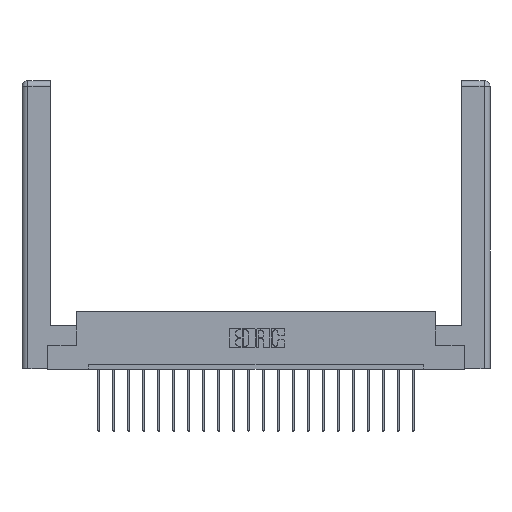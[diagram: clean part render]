
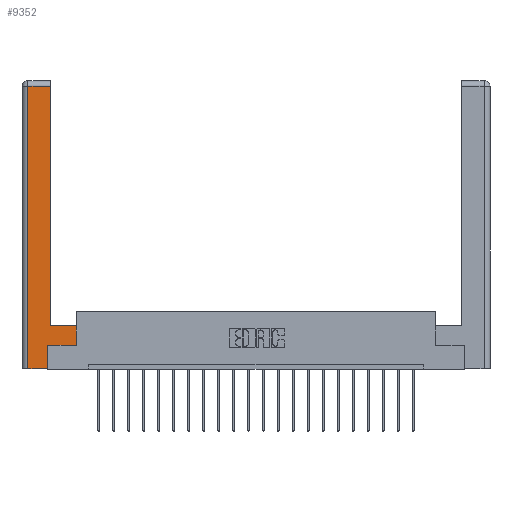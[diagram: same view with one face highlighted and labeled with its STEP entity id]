
A CAD part, top view. The second image highlights one B-rep face of the part: STEP entity #9352.
In plain terms, the highlighted planar face has unit normal (0, 0, 1).
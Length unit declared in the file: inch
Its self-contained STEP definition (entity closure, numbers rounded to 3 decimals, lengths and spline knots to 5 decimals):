
#75 = DIRECTION ( 'NONE',  ( 0., 1., 0. ) ) ;
#248 = VERTEX_POINT ( 'NONE', #835 ) ;
#651 = DIRECTION ( 'NONE',  ( 1., 0., 0. ) ) ;
#835 = CARTESIAN_POINT ( 'NONE',  ( 0.265, 0.245, 0. ) ) ;
#1026 = CARTESIAN_POINT ( 'NONE',  ( 0.295, 3., 0. ) ) ;
#1668 = ORIENTED_EDGE ( 'NONE', *, *, #7298, .T. ) ;
#2332 = CARTESIAN_POINT ( 'NONE',  ( 0.295, 0.45, 0. ) ) ;
#2423 = VERTEX_POINT ( 'NONE', #12963 ) ;
#3326 = CARTESIAN_POINT ( 'NONE',  ( 0.265, 0., 0. ) ) ;
#3584 = LINE ( 'NONE', #17032, #11918 ) ;
#3739 = CARTESIAN_POINT ( 'NONE',  ( 0.0615, 2.94, 0. ) ) ;
#3885 = LINE ( 'NONE', #20429, #16706 ) ;
#3983 = CARTESIAN_POINT ( 'NONE',  ( 0.295, 0.45, 0. ) ) ;
#4080 = ORIENTED_EDGE ( 'NONE', *, *, #11053, .T. ) ;
#4173 = CARTESIAN_POINT ( 'NONE',  ( 0.0615, 0., 0. ) ) ;
#4557 = VECTOR ( 'NONE', #16235, 39.37008 ) ;
#5011 = VERTEX_POINT ( 'NONE', #5076 ) ;
#5012 = CARTESIAN_POINT ( 'NONE',  ( 0., 0., 0. ) ) ;
#5076 = CARTESIAN_POINT ( 'NONE',  ( 0.565, 0.45, 0. ) ) ;
#5267 = AXIS2_PLACEMENT_3D ( 'NONE', #5012, #10126, #20235 ) ;
#5291 = VERTEX_POINT ( 'NONE', #2332 ) ;
#5506 = EDGE_CURVE ( 'NONE', #18912, #248, #3584, .T. ) ;
#5746 = LINE ( 'NONE', #15785, #8893 ) ;
#5751 = DIRECTION ( 'NONE',  ( -1., 0., 0. ) ) ;
#6226 = CARTESIAN_POINT ( 'NONE',  ( 0.0615, 0., 0. ) ) ;
#6699 = LINE ( 'NONE', #6226, #4557 ) ;
#6967 = EDGE_CURVE ( 'NONE', #5011, #5291, #21251, .T. ) ;
#7298 = EDGE_CURVE ( 'NONE', #2423, #18164, #9268, .T. ) ;
#7407 = VECTOR ( 'NONE', #11629, 39.37008 ) ;
#7627 = ORIENTED_EDGE ( 'NONE', *, *, #17752, .T. ) ;
#7664 = ORIENTED_EDGE ( 'NONE', *, *, #5506, .T. ) ;
#8056 = VECTOR ( 'NONE', #17712, 39.37008 ) ;
#8392 = FACE_OUTER_BOUND ( 'NONE', #14338, .T. ) ;
#8604 = LINE ( 'NONE', #1026, #8056 ) ;
#8893 = VECTOR ( 'NONE', #12762, 39.37008 ) ;
#9268 = LINE ( 'NONE', #3739, #15536 ) ;
#9352 = ADVANCED_FACE ( 'NONE', ( #8392 ), #11835, .F. ) ;
#10126 = DIRECTION ( 'NONE',  ( 0., 0., -1. ) ) ;
#10221 = EDGE_CURVE ( 'NONE', #248, #13329, #5746, .T. ) ;
#11053 = EDGE_CURVE ( 'NONE', #5291, #2423, #8604, .T. ) ;
#11629 = DIRECTION ( 'NONE',  ( 0., 1., 0. ) ) ;
#11835 = PLANE ( 'NONE',  #5267 ) ;
#11918 = VECTOR ( 'NONE', #75, 39.37008 ) ;
#12762 = DIRECTION ( 'NONE',  ( 1., 0., 0. ) ) ;
#12963 = CARTESIAN_POINT ( 'NONE',  ( 0.295, 2.94, 0. ) ) ;
#13205 = ORIENTED_EDGE ( 'NONE', *, *, #19686, .T. ) ;
#13329 = VERTEX_POINT ( 'NONE', #17117 ) ;
#14338 = EDGE_LOOP ( 'NONE', ( #4080, #1668, #13205, #7627, #7664, #17806, #17234, #15588 ) ) ;
#14936 = CARTESIAN_POINT ( 'NONE',  ( 0.565, 0.45, 0. ) ) ;
#15370 = DIRECTION ( 'NONE',  ( -1., 0., 0. ) ) ;
#15536 = VECTOR ( 'NONE', #15370, 39.37008 ) ;
#15588 = ORIENTED_EDGE ( 'NONE', *, *, #6967, .T. ) ;
#15785 = CARTESIAN_POINT ( 'NONE',  ( 0.565, 0.245, 0. ) ) ;
#16235 = DIRECTION ( 'NONE',  ( 0., -1., 0. ) ) ;
#16336 = VECTOR ( 'NONE', #5751, 39.37008 ) ;
#16706 = VECTOR ( 'NONE', #651, 39.37008 ) ;
#17032 = CARTESIAN_POINT ( 'NONE',  ( 0.265, 0.245, 0. ) ) ;
#17117 = CARTESIAN_POINT ( 'NONE',  ( 0.565, 0.245, 0. ) ) ;
#17234 = ORIENTED_EDGE ( 'NONE', *, *, #20977, .T. ) ;
#17255 = VERTEX_POINT ( 'NONE', #4173 ) ;
#17712 = DIRECTION ( 'NONE',  ( 0., 1., 0. ) ) ;
#17752 = EDGE_CURVE ( 'NONE', #17255, #18912, #3885, .T. ) ;
#17806 = ORIENTED_EDGE ( 'NONE', *, *, #10221, .T. ) ;
#18112 = LINE ( 'NONE', #14936, #7407 ) ;
#18164 = VERTEX_POINT ( 'NONE', #21493 ) ;
#18912 = VERTEX_POINT ( 'NONE', #3326 ) ;
#19686 = EDGE_CURVE ( 'NONE', #18164, #17255, #6699, .T. ) ;
#20235 = DIRECTION ( 'NONE',  ( -1., 0., 0. ) ) ;
#20429 = CARTESIAN_POINT ( 'NONE',  ( 0.265, 0., 0. ) ) ;
#20977 = EDGE_CURVE ( 'NONE', #13329, #5011, #18112, .T. ) ;
#21251 = LINE ( 'NONE', #3983, #16336 ) ;
#21493 = CARTESIAN_POINT ( 'NONE',  ( 0.0615, 2.94, 0. ) ) ;
